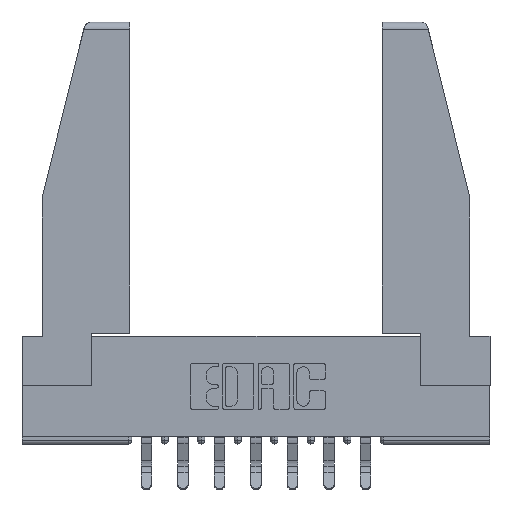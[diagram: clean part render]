
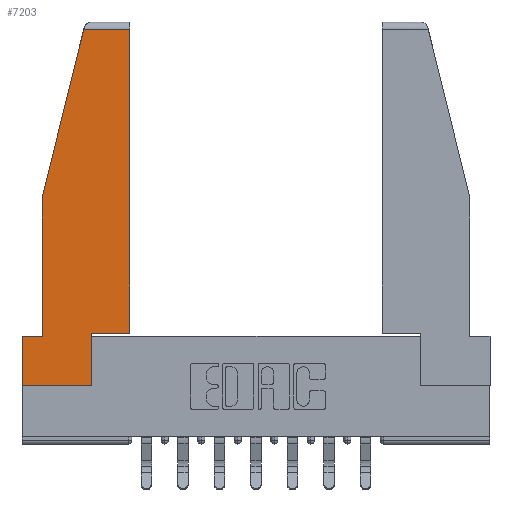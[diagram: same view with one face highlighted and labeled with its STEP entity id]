
A CAD part, top view. The second image highlights one B-rep face of the part: STEP entity #7203.
In plain terms, the highlighted planar face has unit normal (0, 0, 1).
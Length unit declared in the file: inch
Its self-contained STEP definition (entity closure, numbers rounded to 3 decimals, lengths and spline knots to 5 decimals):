
#116 = DIRECTION ( 'NONE',  ( 1., 0., 0. ) ) ;
#586 = VECTOR ( 'NONE', #14406, 39.37008 ) ;
#967 = EDGE_LOOP ( 'NONE', ( #11705, #2160, #7462, #13647, #13730, #6417, #14038, #7374, #6846 ) ) ;
#1379 = DIRECTION ( 'NONE',  ( 0., 1., 0. ) ) ;
#1414 = CARTESIAN_POINT ( 'NONE',  ( 0.297, 0.223, 0. ) ) ;
#1425 = VERTEX_POINT ( 'NONE', #8532 ) ;
#1428 = CARTESIAN_POINT ( 'NONE',  ( 0., 0., 0. ) ) ;
#1615 = VERTEX_POINT ( 'NONE', #5263 ) ;
#1680 = EDGE_CURVE ( 'NONE', #3962, #6532, #9013, .T. ) ;
#1719 = EDGE_CURVE ( 'NONE', #1615, #3962, #8635, .T. ) ;
#1798 = CARTESIAN_POINT ( 'NONE',  ( 0.271, 1.55, 0. ) ) ;
#1846 = CARTESIAN_POINT ( 'NONE',  ( 0.297, 0.223, 0. ) ) ;
#1894 = PLANE ( 'NONE',  #11614 ) ;
#2160 = ORIENTED_EDGE ( 'NONE', *, *, #5819, .T. ) ;
#2581 = CARTESIAN_POINT ( 'NONE',  ( 0.297, 0., 0. ) ) ;
#2734 = DIRECTION ( 'NONE',  ( 0., 1., 0. ) ) ;
#2959 = CARTESIAN_POINT ( 'NONE',  ( 0., 0., 0. ) ) ;
#3120 = CARTESIAN_POINT ( 'NONE',  ( 0., 0.21, 0. ) ) ;
#3509 = CARTESIAN_POINT ( 'NONE',  ( 0., 1.52, 0. ) ) ;
#3548 = LINE ( 'NONE', #3120, #586 ) ;
#3591 = VERTEX_POINT ( 'NONE', #12706 ) ;
#3829 = VERTEX_POINT ( 'NONE', #7228 ) ;
#3909 = FACE_OUTER_BOUND ( 'NONE', #967, .T. ) ;
#3962 = VERTEX_POINT ( 'NONE', #7041 ) ;
#4303 = LINE ( 'NONE', #9468, #5365 ) ;
#4525 = DIRECTION ( 'NONE',  ( -1., 0., 0. ) ) ;
#5222 = VERTEX_POINT ( 'NONE', #1846 ) ;
#5263 = CARTESIAN_POINT ( 'NONE',  ( 0.086, 0.8, 0. ) ) ;
#5365 = VECTOR ( 'NONE', #2734, 39.37008 ) ;
#5651 = DIRECTION ( 'NONE',  ( 1., 0., 0. ) ) ;
#5819 = EDGE_CURVE ( 'NONE', #14323, #3829, #10316, .T. ) ;
#6018 = EDGE_CURVE ( 'NONE', #3591, #14323, #4303, .T. ) ;
#6276 = VECTOR ( 'NONE', #1379, 39.37008 ) ;
#6417 = ORIENTED_EDGE ( 'NONE', *, *, #12361, .T. ) ;
#6532 = VERTEX_POINT ( 'NONE', #10640 ) ;
#6665 = EDGE_CURVE ( 'NONE', #3829, #1615, #10974, .T. ) ;
#6751 = CARTESIAN_POINT ( 'NONE',  ( 0., 0.21, 0. ) ) ;
#6846 = ORIENTED_EDGE ( 'NONE', *, *, #8598, .T. ) ;
#6950 = VECTOR ( 'NONE', #4525, 39.37008 ) ;
#7041 = CARTESIAN_POINT ( 'NONE',  ( 0.086, 0.21, 0. ) ) ;
#7160 = LINE ( 'NONE', #2581, #6276 ) ;
#7203 = ADVANCED_FACE ( 'NONE', ( #3909 ), #1894, .T. ) ;
#7228 = CARTESIAN_POINT ( 'NONE',  ( 0.2636, 1.52, 0. ) ) ;
#7374 = ORIENTED_EDGE ( 'NONE', *, *, #11449, .T. ) ;
#7462 = ORIENTED_EDGE ( 'NONE', *, *, #6665, .T. ) ;
#7711 = EDGE_CURVE ( 'NONE', #1425, #13521, #8124, .T. ) ;
#8124 = LINE ( 'NONE', #1428, #8321 ) ;
#8321 = VECTOR ( 'NONE', #116, 39.37008 ) ;
#8532 = CARTESIAN_POINT ( 'NONE',  ( 0., 0., 0. ) ) ;
#8598 = EDGE_CURVE ( 'NONE', #5222, #3591, #9375, .T. ) ;
#8635 = LINE ( 'NONE', #8743, #13741 ) ;
#8743 = CARTESIAN_POINT ( 'NONE',  ( 0.086, 0.8, 0. ) ) ;
#9013 = LINE ( 'NONE', #6751, #13380 ) ;
#9063 = VECTOR ( 'NONE', #9605, 39.37008 ) ;
#9375 = LINE ( 'NONE', #1414, #13205 ) ;
#9468 = CARTESIAN_POINT ( 'NONE',  ( 0.461, 0.223, 0. ) ) ;
#9604 = DIRECTION ( 'NONE',  ( 0., 0., 1. ) ) ;
#9605 = DIRECTION ( 'NONE',  ( -0.239, -0.971, 0. ) ) ;
#9989 = DIRECTION ( 'NONE',  ( 0., -1., 0. ) ) ;
#10197 = CARTESIAN_POINT ( 'NONE',  ( 0.297, 0., 0. ) ) ;
#10316 = LINE ( 'NONE', #3509, #6950 ) ;
#10640 = CARTESIAN_POINT ( 'NONE',  ( 0., 0.21, 0. ) ) ;
#10974 = LINE ( 'NONE', #1798, #9063 ) ;
#11449 = EDGE_CURVE ( 'NONE', #13521, #5222, #7160, .T. ) ;
#11599 = CARTESIAN_POINT ( 'NONE',  ( 0.461, 1.52, 0. ) ) ;
#11614 = AXIS2_PLACEMENT_3D ( 'NONE', #2959, #9604, #11936 ) ;
#11705 = ORIENTED_EDGE ( 'NONE', *, *, #6018, .T. ) ;
#11936 = DIRECTION ( 'NONE',  ( 1., 0., 0. ) ) ;
#12361 = EDGE_CURVE ( 'NONE', #6532, #1425, #3548, .T. ) ;
#12392 = DIRECTION ( 'NONE',  ( -1., 0., 0. ) ) ;
#12706 = CARTESIAN_POINT ( 'NONE',  ( 0.461, 0.223, 0. ) ) ;
#13205 = VECTOR ( 'NONE', #5651, 39.37008 ) ;
#13380 = VECTOR ( 'NONE', #12392, 39.37008 ) ;
#13521 = VERTEX_POINT ( 'NONE', #10197 ) ;
#13647 = ORIENTED_EDGE ( 'NONE', *, *, #1719, .T. ) ;
#13730 = ORIENTED_EDGE ( 'NONE', *, *, #1680, .T. ) ;
#13741 = VECTOR ( 'NONE', #9989, 39.37008 ) ;
#14038 = ORIENTED_EDGE ( 'NONE', *, *, #7711, .T. ) ;
#14323 = VERTEX_POINT ( 'NONE', #11599 ) ;
#14406 = DIRECTION ( 'NONE',  ( 0., -1., 0. ) ) ;
